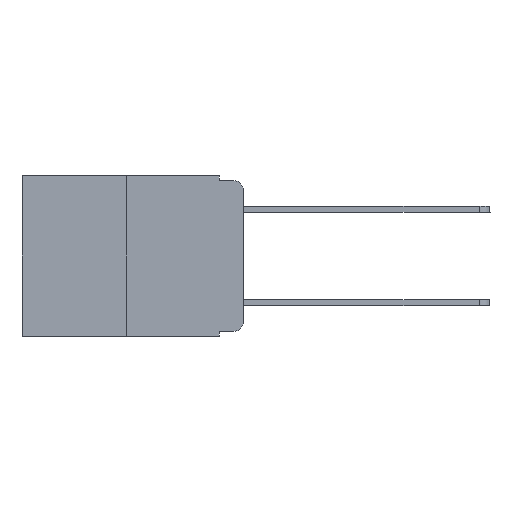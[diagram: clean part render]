
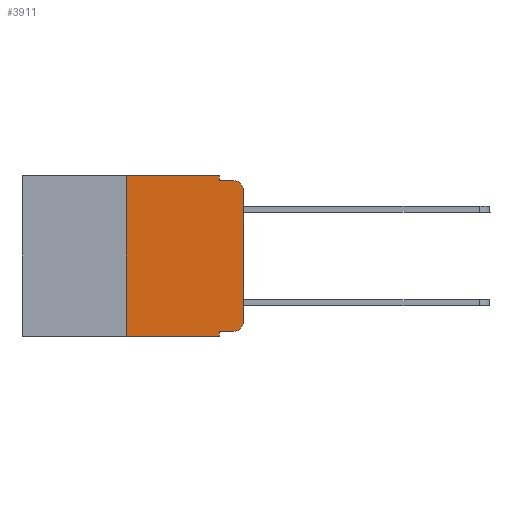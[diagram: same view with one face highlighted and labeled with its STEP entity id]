
A CAD part, left-side view. The second image highlights one B-rep face of the part: STEP entity #3911.
In plain terms, the highlighted planar face has unit normal (-1, 0, 0).
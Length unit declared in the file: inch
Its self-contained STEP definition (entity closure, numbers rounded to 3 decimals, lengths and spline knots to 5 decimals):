
#398 = VERTEX_POINT ( 'NONE', #12881 ) ;
#509 = CARTESIAN_POINT ( 'NONE',  ( 0., 0.473, 0. ) ) ;
#573 = VECTOR ( 'NONE', #8293, 39.37008 ) ;
#816 = LINE ( 'NONE', #1240, #19606 ) ;
#1240 = CARTESIAN_POINT ( 'NONE',  ( 0., 0.051, -0.01 ) ) ;
#1314 = EDGE_CURVE ( 'NONE', #14391, #24586, #2420, .T. ) ;
#1769 = CIRCLE ( 'NONE', #15962, 0.02 ) ;
#2420 = LINE ( 'NONE', #11958, #573 ) ;
#2610 = VECTOR ( 'NONE', #4510, 39.37008 ) ;
#2625 = FACE_OUTER_BOUND ( 'NONE', #20176, .T. ) ;
#2789 = EDGE_CURVE ( 'NONE', #4535, #14391, #16248, .T. ) ;
#2845 = VERTEX_POINT ( 'NONE', #16465 ) ;
#2889 = EDGE_CURVE ( 'NONE', #7679, #4535, #17132, .T. ) ;
#3309 = VERTEX_POINT ( 'NONE', #12905 ) ;
#3316 = DIRECTION ( 'NONE',  ( -1., 0., 0. ) ) ;
#3376 = AXIS2_PLACEMENT_3D ( 'NONE', #8608, #16714, #20517 ) ;
#3683 = VERTEX_POINT ( 'NONE', #15866 ) ;
#3911 = ADVANCED_FACE ( 'NONE', ( #2625 ), #18683, .F. ) ;
#4422 = ORIENTED_EDGE ( 'NONE', *, *, #6195, .F. ) ;
#4510 = DIRECTION ( 'NONE',  ( 0., 0., -1. ) ) ;
#4535 = VERTEX_POINT ( 'NONE', #6245 ) ;
#4638 = CARTESIAN_POINT ( 'NONE',  ( 0., 0., -0.313 ) ) ;
#4807 = CARTESIAN_POINT ( 'NONE',  ( 0., 0.25, 0. ) ) ;
#4956 = ORIENTED_EDGE ( 'NONE', *, *, #11806, .T. ) ;
#5172 = EDGE_CURVE ( 'NONE', #22557, #3683, #11937, .T. ) ;
#5291 = ORIENTED_EDGE ( 'NONE', *, *, #1314, .T. ) ;
#5379 = CARTESIAN_POINT ( 'NONE',  ( 0., 0.051, 0. ) ) ;
#5580 = LINE ( 'NONE', #15163, #22537 ) ;
#6195 = EDGE_CURVE ( 'NONE', #398, #2845, #816, .T. ) ;
#6245 = CARTESIAN_POINT ( 'NONE',  ( 0., 0.02, -0.333 ) ) ;
#6312 = CARTESIAN_POINT ( 'NONE',  ( 0., 0.051, 0. ) ) ;
#6503 = VECTOR ( 'NONE', #20658, 39.37008 ) ;
#6790 = DIRECTION ( 'NONE',  ( 0., 0., -1. ) ) ;
#7576 = VECTOR ( 'NONE', #21884, 39.37008 ) ;
#7679 = VERTEX_POINT ( 'NONE', #7730 ) ;
#7730 = CARTESIAN_POINT ( 'NONE',  ( 0., 0.051, -0.333 ) ) ;
#8293 = DIRECTION ( 'NONE',  ( 0., 0., 1. ) ) ;
#8602 = CARTESIAN_POINT ( 'NONE',  ( 0., 0.473, 0. ) ) ;
#8608 = CARTESIAN_POINT ( 'NONE',  ( 0., 0.02, -0.313 ) ) ;
#8647 = LINE ( 'NONE', #4807, #6503 ) ;
#10894 = DIRECTION ( 'NONE',  ( 0., -1., 0. ) ) ;
#11806 = EDGE_CURVE ( 'NONE', #24586, #2845, #1769, .T. ) ;
#11937 = LINE ( 'NONE', #12020, #7576 ) ;
#11958 = CARTESIAN_POINT ( 'NONE',  ( 0., 0., 0. ) ) ;
#12020 = CARTESIAN_POINT ( 'NONE',  ( 0., 0.473, -0.343 ) ) ;
#12881 = CARTESIAN_POINT ( 'NONE',  ( 0., 0.051, -0.01 ) ) ;
#12905 = CARTESIAN_POINT ( 'NONE',  ( 0., 0.25, 0. ) ) ;
#13239 = ORIENTED_EDGE ( 'NONE', *, *, #13711, .F. ) ;
#13518 = ORIENTED_EDGE ( 'NONE', *, *, #2889, .T. ) ;
#13711 = EDGE_CURVE ( 'NONE', #16639, #398, #23545, .T. ) ;
#14391 = VERTEX_POINT ( 'NONE', #4638 ) ;
#15163 = CARTESIAN_POINT ( 'NONE',  ( 0., 0.051, 0. ) ) ;
#15623 = VECTOR ( 'NONE', #10894, 39.37008 ) ;
#15809 = EDGE_CURVE ( 'NONE', #22557, #3309, #8647, .T. ) ;
#15866 = CARTESIAN_POINT ( 'NONE',  ( 0., 0.051, -0.343 ) ) ;
#15962 = AXIS2_PLACEMENT_3D ( 'NONE', #19089, #3316, #19162 ) ;
#16248 = CIRCLE ( 'NONE', #3376, 0.02 ) ;
#16266 = EDGE_CURVE ( 'NONE', #3309, #16639, #16338, .T. ) ;
#16338 = LINE ( 'NONE', #509, #22810 ) ;
#16465 = CARTESIAN_POINT ( 'NONE',  ( 0., 0.02, -0.01 ) ) ;
#16607 = CARTESIAN_POINT ( 'NONE',  ( 0., 0.25, -0.343 ) ) ;
#16639 = VERTEX_POINT ( 'NONE', #5379 ) ;
#16714 = DIRECTION ( 'NONE',  ( -1., 0., 0. ) ) ;
#17132 = LINE ( 'NONE', #24725, #15623 ) ;
#18185 = ORIENTED_EDGE ( 'NONE', *, *, #2789, .T. ) ;
#18302 = ORIENTED_EDGE ( 'NONE', *, *, #16266, .F. ) ;
#18683 = PLANE ( 'NONE',  #20742 ) ;
#19089 = CARTESIAN_POINT ( 'NONE',  ( 0., 0.02, -0.03 ) ) ;
#19140 = EDGE_CURVE ( 'NONE', #7679, #3683, #5580, .T. ) ;
#19162 = DIRECTION ( 'NONE',  ( 0., 0., -1. ) ) ;
#19606 = VECTOR ( 'NONE', #24663, 39.37008 ) ;
#19780 = ORIENTED_EDGE ( 'NONE', *, *, #15809, .F. ) ;
#20176 = EDGE_LOOP ( 'NONE', ( #5291, #4956, #4422, #13239, #18302, #19780, #23611, #20731, #13518, #18185 ) ) ;
#20506 = DIRECTION ( 'NONE',  ( 1., 0., 0. ) ) ;
#20517 = DIRECTION ( 'NONE',  ( 0., 0., -1. ) ) ;
#20658 = DIRECTION ( 'NONE',  ( 0., 0., 1. ) ) ;
#20731 = ORIENTED_EDGE ( 'NONE', *, *, #19140, .F. ) ;
#20742 = AXIS2_PLACEMENT_3D ( 'NONE', #8602, #20506, #6790 ) ;
#21789 = CARTESIAN_POINT ( 'NONE',  ( 0., 0., -0.03 ) ) ;
#21884 = DIRECTION ( 'NONE',  ( 0., -1., 0. ) ) ;
#22184 = DIRECTION ( 'NONE',  ( 0., -1., 0. ) ) ;
#22537 = VECTOR ( 'NONE', #24703, 39.37008 ) ;
#22557 = VERTEX_POINT ( 'NONE', #16607 ) ;
#22810 = VECTOR ( 'NONE', #22184, 39.37008 ) ;
#23545 = LINE ( 'NONE', #6312, #2610 ) ;
#23611 = ORIENTED_EDGE ( 'NONE', *, *, #5172, .T. ) ;
#24586 = VERTEX_POINT ( 'NONE', #21789 ) ;
#24663 = DIRECTION ( 'NONE',  ( 0., -1., 0. ) ) ;
#24703 = DIRECTION ( 'NONE',  ( 0., 0., -1. ) ) ;
#24725 = CARTESIAN_POINT ( 'NONE',  ( 0., 0.051, -0.333 ) ) ;
